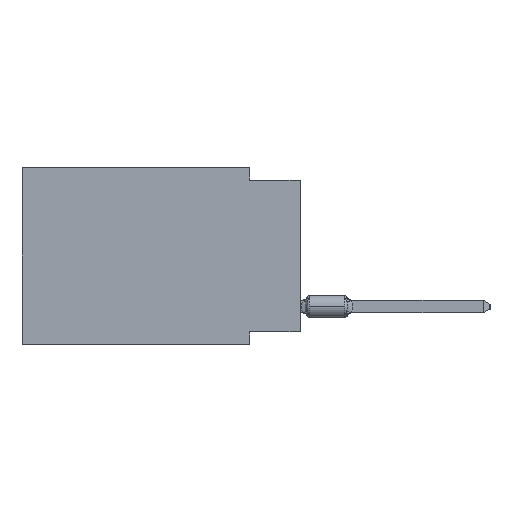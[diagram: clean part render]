
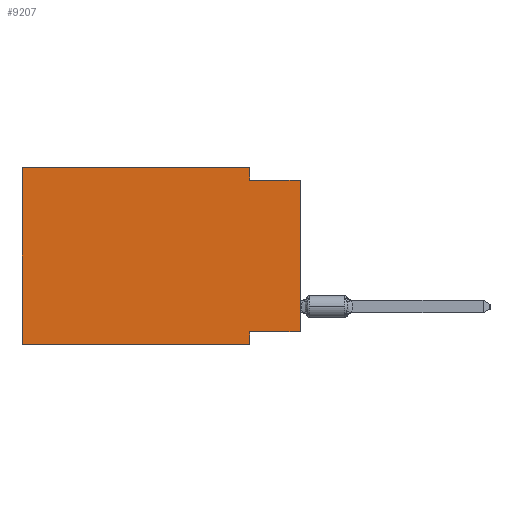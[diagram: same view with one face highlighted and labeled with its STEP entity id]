
A CAD part, left-side view. The second image highlights one B-rep face of the part: STEP entity #9207.
In plain terms, the highlighted planar face has unit normal (-1, 0, 0).
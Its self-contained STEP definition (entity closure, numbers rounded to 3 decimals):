
#1213 = CARTESIAN_POINT ( 'NONE',  ( 0., 0., -0.635 ) ) ;
#1382 = LINE ( 'NONE', #45907, #35394 ) ;
#1620 = EDGE_LOOP ( 'NONE', ( #33287, #2450, #12679, #14453, #37524, #44011, #10038, #32796 ) ) ;
#1750 = LINE ( 'NONE', #11980, #17611 ) ;
#2450 = ORIENTED_EDGE ( 'NONE', *, *, #25800, .F. ) ;
#2939 = DIRECTION ( 'NONE',  ( 0., 0., 1. ) ) ;
#3255 = CARTESIAN_POINT ( 'NONE',  ( 0., 2.54, 0. ) ) ;
#6619 = CARTESIAN_POINT ( 'NONE',  ( 0., 2.54, -8.255 ) ) ;
#9207 = ADVANCED_FACE ( 'NONE', ( #47978 ), #17815, .F. ) ;
#9224 = DIRECTION ( 'NONE',  ( 0., -1., 0. ) ) ;
#9583 = DIRECTION ( 'NONE',  ( 0., 1., 0. ) ) ;
#9803 = CARTESIAN_POINT ( 'NONE',  ( 0., 2.54, 0. ) ) ;
#9877 = VECTOR ( 'NONE', #9583, 1000. ) ;
#10038 = ORIENTED_EDGE ( 'NONE', *, *, #38196, .F. ) ;
#10300 = EDGE_CURVE ( 'NONE', #41621, #39252, #20990, .T. ) ;
#10511 = DIRECTION ( 'NONE',  ( 1., 0., 0. ) ) ;
#10831 = VERTEX_POINT ( 'NONE', #13873 ) ;
#11980 = CARTESIAN_POINT ( 'NONE',  ( 0., 13.97, 0. ) ) ;
#12679 = ORIENTED_EDGE ( 'NONE', *, *, #10300, .F. ) ;
#13873 = CARTESIAN_POINT ( 'NONE',  ( 0., 13.97, -8.89 ) ) ;
#14453 = ORIENTED_EDGE ( 'NONE', *, *, #40848, .F. ) ;
#17611 = VECTOR ( 'NONE', #37746, 1000. ) ;
#17815 = PLANE ( 'NONE',  #37224 ) ;
#18289 = DIRECTION ( 'NONE',  ( 0., 0., -1. ) ) ;
#20710 = VECTOR ( 'NONE', #47378, 1000. ) ;
#20796 = LINE ( 'NONE', #28349, #27911 ) ;
#20990 = LINE ( 'NONE', #9803, #30961 ) ;
#21104 = CARTESIAN_POINT ( 'NONE',  ( 0., 2.54, -8.89 ) ) ;
#21914 = CARTESIAN_POINT ( 'NONE',  ( 0., 0., -0.635 ) ) ;
#24314 = EDGE_CURVE ( 'NONE', #10831, #46069, #28486, .T. ) ;
#25800 = EDGE_CURVE ( 'NONE', #39252, #41068, #27249, .T. ) ;
#27249 = LINE ( 'NONE', #1213, #30070 ) ;
#27646 = VECTOR ( 'NONE', #2939, 1000. ) ;
#27911 = VECTOR ( 'NONE', #32953, 1000. ) ;
#27934 = LINE ( 'NONE', #21104, #20710 ) ;
#28083 = CARTESIAN_POINT ( 'NONE',  ( 0., 0., -8.255 ) ) ;
#28288 = CARTESIAN_POINT ( 'NONE',  ( 0., 0., -8.255 ) ) ;
#28349 = CARTESIAN_POINT ( 'NONE',  ( 0., 0., 0. ) ) ;
#28486 = LINE ( 'NONE', #44045, #27646 ) ;
#30070 = VECTOR ( 'NONE', #9224, 1000. ) ;
#30959 = VERTEX_POINT ( 'NONE', #6619 ) ;
#30961 = VECTOR ( 'NONE', #32423, 1000. ) ;
#32423 = DIRECTION ( 'NONE',  ( 0., 0., -1. ) ) ;
#32796 = ORIENTED_EDGE ( 'NONE', *, *, #40614, .F. ) ;
#32953 = DIRECTION ( 'NONE',  ( 0., 0., 1. ) ) ;
#33287 = ORIENTED_EDGE ( 'NONE', *, *, #43361, .T. ) ;
#34429 = CARTESIAN_POINT ( 'NONE',  ( 0., 2.54, -8.89 ) ) ;
#35394 = VECTOR ( 'NONE', #42244, 1000. ) ;
#36233 = VERTEX_POINT ( 'NONE', #28288 ) ;
#36539 = CARTESIAN_POINT ( 'NONE',  ( 0., 13.97, 0. ) ) ;
#37224 = AXIS2_PLACEMENT_3D ( 'NONE', #36539, #10511, #18289 ) ;
#37524 = ORIENTED_EDGE ( 'NONE', *, *, #24314, .F. ) ;
#37746 = DIRECTION ( 'NONE',  ( 0., -1., 0. ) ) ;
#38196 = EDGE_CURVE ( 'NONE', #30959, #41474, #27934, .T. ) ;
#39252 = VERTEX_POINT ( 'NONE', #47272 ) ;
#40614 = EDGE_CURVE ( 'NONE', #36233, #30959, #47040, .T. ) ;
#40848 = EDGE_CURVE ( 'NONE', #46069, #41621, #1750, .T. ) ;
#41068 = VERTEX_POINT ( 'NONE', #21914 ) ;
#41474 = VERTEX_POINT ( 'NONE', #34429 ) ;
#41621 = VERTEX_POINT ( 'NONE', #3255 ) ;
#41951 = CARTESIAN_POINT ( 'NONE',  ( 0., 13.97, 0. ) ) ;
#42244 = DIRECTION ( 'NONE',  ( 0., -1., 0. ) ) ;
#43361 = EDGE_CURVE ( 'NONE', #36233, #41068, #20796, .T. ) ;
#44011 = ORIENTED_EDGE ( 'NONE', *, *, #45786, .T. ) ;
#44045 = CARTESIAN_POINT ( 'NONE',  ( 0., 13.97, 0. ) ) ;
#45786 = EDGE_CURVE ( 'NONE', #10831, #41474, #1382, .T. ) ;
#45907 = CARTESIAN_POINT ( 'NONE',  ( 0., 13.97, -8.89 ) ) ;
#46069 = VERTEX_POINT ( 'NONE', #41951 ) ;
#47040 = LINE ( 'NONE', #28083, #9877 ) ;
#47272 = CARTESIAN_POINT ( 'NONE',  ( 0., 2.54, -0.635 ) ) ;
#47378 = DIRECTION ( 'NONE',  ( 0., 0., -1. ) ) ;
#47978 = FACE_OUTER_BOUND ( 'NONE', #1620, .T. ) ;
